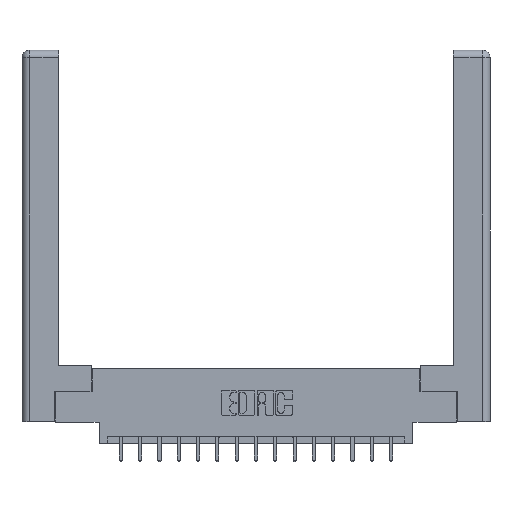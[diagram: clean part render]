
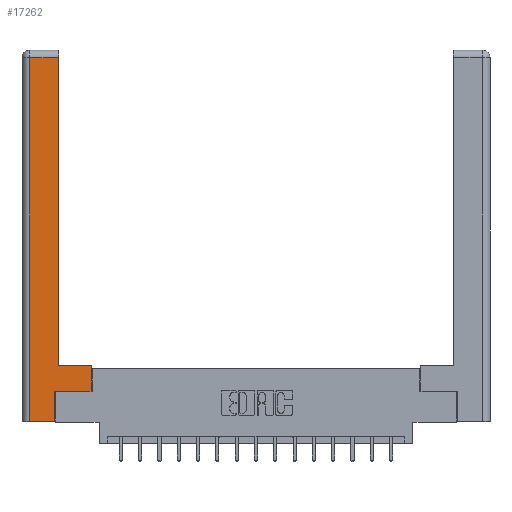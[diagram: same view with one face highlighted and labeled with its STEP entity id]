
A CAD part, top view. The second image highlights one B-rep face of the part: STEP entity #17262.
In plain terms, the highlighted planar face has unit normal (0, 0, 1).
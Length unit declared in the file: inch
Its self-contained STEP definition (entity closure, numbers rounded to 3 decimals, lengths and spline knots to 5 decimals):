
#132 = PLANE ( 'NONE',  #4940 ) ;
#255 = VERTEX_POINT ( 'NONE', #16616 ) ;
#316 = DIRECTION ( 'NONE',  ( 0., 0., -1. ) ) ;
#507 = EDGE_CURVE ( 'NONE', #11208, #8051, #16486, .T. ) ;
#1070 = ORIENTED_EDGE ( 'NONE', *, *, #12685, .T. ) ;
#1173 = CARTESIAN_POINT ( 'NONE',  ( 0.565, 0.245, 0. ) ) ;
#1590 = DIRECTION ( 'NONE',  ( -1., 0., 0. ) ) ;
#1851 = ORIENTED_EDGE ( 'NONE', *, *, #15225, .T. ) ;
#2129 = CARTESIAN_POINT ( 'NONE',  ( 0.0615, 0., 0. ) ) ;
#2330 = CARTESIAN_POINT ( 'NONE',  ( 0.0615, 0., 0. ) ) ;
#2493 = CARTESIAN_POINT ( 'NONE',  ( 0.265, 0., 0. ) ) ;
#2525 = VERTEX_POINT ( 'NONE', #12571 ) ;
#2596 = VERTEX_POINT ( 'NONE', #11359 ) ;
#3012 = LINE ( 'NONE', #5265, #15324 ) ;
#3280 = CARTESIAN_POINT ( 'NONE',  ( 0.0615, 2.94, 0. ) ) ;
#3468 = VECTOR ( 'NONE', #7821, 39.37008 ) ;
#4928 = FACE_OUTER_BOUND ( 'NONE', #5425, .T. ) ;
#4940 = AXIS2_PLACEMENT_3D ( 'NONE', #7201, #316, #1590 ) ;
#5265 = CARTESIAN_POINT ( 'NONE',  ( 0.0615, 2.94, 0. ) ) ;
#5425 = EDGE_LOOP ( 'NONE', ( #1851, #12935, #7017, #9231, #1070, #14486, #13070, #10758 ) ) ;
#6708 = CARTESIAN_POINT ( 'NONE',  ( 0.565, 0.45, 0. ) ) ;
#7017 = ORIENTED_EDGE ( 'NONE', *, *, #507, .T. ) ;
#7201 = CARTESIAN_POINT ( 'NONE',  ( 0., 0., 0. ) ) ;
#7242 = LINE ( 'NONE', #1173, #17858 ) ;
#7320 = LINE ( 'NONE', #16725, #14915 ) ;
#7538 = LINE ( 'NONE', #16295, #3468 ) ;
#7821 = DIRECTION ( 'NONE',  ( -1., 0., 0. ) ) ;
#7951 = EDGE_CURVE ( 'NONE', #9508, #2596, #7242, .T. ) ;
#8051 = VERTEX_POINT ( 'NONE', #2330 ) ;
#8058 = CARTESIAN_POINT ( 'NONE',  ( 0.265, 0.245, 0. ) ) ;
#8253 = VECTOR ( 'NONE', #12138, 39.37008 ) ;
#8683 = LINE ( 'NONE', #10579, #8253 ) ;
#8944 = LINE ( 'NONE', #11274, #17621 ) ;
#9231 = ORIENTED_EDGE ( 'NONE', *, *, #11201, .T. ) ;
#9265 = DIRECTION ( 'NONE',  ( 1., 0., 0. ) ) ;
#9508 = VERTEX_POINT ( 'NONE', #8058 ) ;
#10062 = VERTEX_POINT ( 'NONE', #2493 ) ;
#10579 = CARTESIAN_POINT ( 'NONE',  ( 0.295, 3., 0. ) ) ;
#10758 = ORIENTED_EDGE ( 'NONE', *, *, #10888, .T. ) ;
#10888 = EDGE_CURVE ( 'NONE', #12229, #2525, #7538, .T. ) ;
#11201 = EDGE_CURVE ( 'NONE', #8051, #10062, #7320, .T. ) ;
#11208 = VERTEX_POINT ( 'NONE', #3280 ) ;
#11274 = CARTESIAN_POINT ( 'NONE',  ( 0.565, 0.45, 0. ) ) ;
#11359 = CARTESIAN_POINT ( 'NONE',  ( 0.565, 0.245, 0. ) ) ;
#11443 = DIRECTION ( 'NONE',  ( 1., 0., 0. ) ) ;
#12138 = DIRECTION ( 'NONE',  ( 0., 1., 0. ) ) ;
#12147 = VECTOR ( 'NONE', #12244, 39.37008 ) ;
#12229 = VERTEX_POINT ( 'NONE', #6708 ) ;
#12238 = EDGE_CURVE ( 'NONE', #255, #11208, #3012, .T. ) ;
#12244 = DIRECTION ( 'NONE',  ( 0., -1., 0. ) ) ;
#12246 = DIRECTION ( 'NONE',  ( -1., 0., 0. ) ) ;
#12571 = CARTESIAN_POINT ( 'NONE',  ( 0.295, 0.45, 0. ) ) ;
#12685 = EDGE_CURVE ( 'NONE', #10062, #9508, #13319, .T. ) ;
#12935 = ORIENTED_EDGE ( 'NONE', *, *, #12238, .T. ) ;
#13070 = ORIENTED_EDGE ( 'NONE', *, *, #14266, .T. ) ;
#13319 = LINE ( 'NONE', #14515, #15093 ) ;
#14266 = EDGE_CURVE ( 'NONE', #2596, #12229, #8944, .T. ) ;
#14486 = ORIENTED_EDGE ( 'NONE', *, *, #7951, .T. ) ;
#14515 = CARTESIAN_POINT ( 'NONE',  ( 0.265, 0.245, 0. ) ) ;
#14915 = VECTOR ( 'NONE', #11443, 39.37008 ) ;
#15093 = VECTOR ( 'NONE', #16057, 39.37008 ) ;
#15225 = EDGE_CURVE ( 'NONE', #2525, #255, #8683, .T. ) ;
#15324 = VECTOR ( 'NONE', #12246, 39.37008 ) ;
#16057 = DIRECTION ( 'NONE',  ( 0., 1., 0. ) ) ;
#16295 = CARTESIAN_POINT ( 'NONE',  ( 0.295, 0.45, 0. ) ) ;
#16486 = LINE ( 'NONE', #2129, #12147 ) ;
#16616 = CARTESIAN_POINT ( 'NONE',  ( 0.295, 2.94, 0. ) ) ;
#16725 = CARTESIAN_POINT ( 'NONE',  ( 0.265, 0., 0. ) ) ;
#16926 = DIRECTION ( 'NONE',  ( 0., 1., 0. ) ) ;
#17262 = ADVANCED_FACE ( 'NONE', ( #4928 ), #132, .F. ) ;
#17621 = VECTOR ( 'NONE', #16926, 39.37008 ) ;
#17858 = VECTOR ( 'NONE', #9265, 39.37008 ) ;
